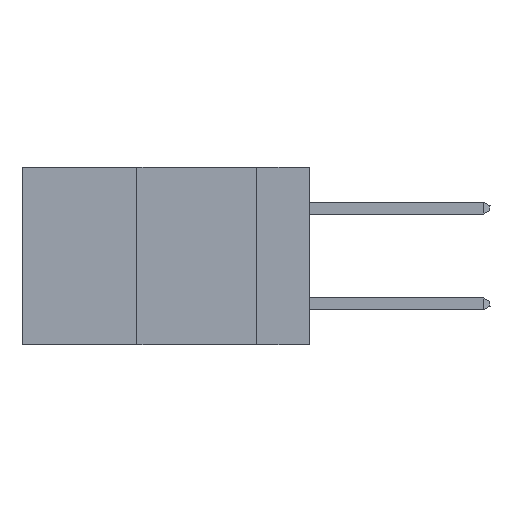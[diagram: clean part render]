
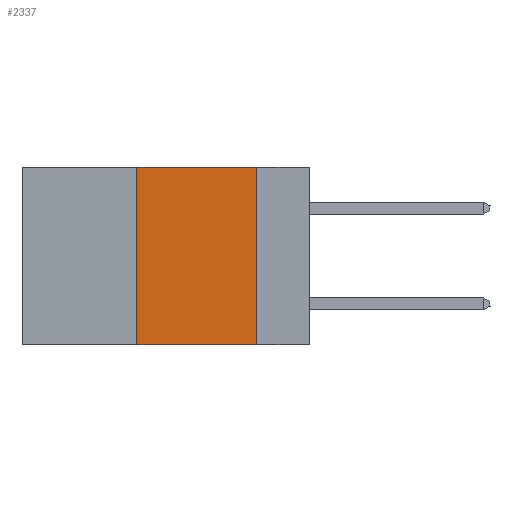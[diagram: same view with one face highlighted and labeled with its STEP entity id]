
A CAD part, left-side view. The second image highlights one B-rep face of the part: STEP entity #2337.
In plain terms, the highlighted planar face has unit normal (-1, 0, 0).
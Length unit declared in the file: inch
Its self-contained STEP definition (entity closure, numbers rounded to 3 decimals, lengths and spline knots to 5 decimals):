
#661 = CARTESIAN_POINT ( 'NONE',  ( 0., 0.36, -0.37 ) ) ;
#684 = VERTEX_POINT ( 'NONE', #33528 ) ;
#2337 = ADVANCED_FACE ( 'NONE', ( #24052 ), #7334, .F. ) ;
#2717 = CARTESIAN_POINT ( 'NONE',  ( 0., 0.6, 0. ) ) ;
#2844 = VECTOR ( 'NONE', #7003, 39.37008 ) ;
#3004 = EDGE_CURVE ( 'NONE', #35442, #684, #9142, .T. ) ;
#4611 = DIRECTION ( 'NONE',  ( 1., 0., 0. ) ) ;
#5510 = CARTESIAN_POINT ( 'NONE',  ( 0., 0.11, 0. ) ) ;
#5900 = EDGE_LOOP ( 'NONE', ( #15593, #10784, #30600, #32843 ) ) ;
#7003 = DIRECTION ( 'NONE',  ( 0., -1., 0. ) ) ;
#7334 = PLANE ( 'NONE',  #17374 ) ;
#9142 = LINE ( 'NONE', #5510, #30997 ) ;
#9614 = EDGE_CURVE ( 'NONE', #21436, #35442, #11652, .T. ) ;
#9817 = EDGE_CURVE ( 'NONE', #29942, #684, #22543, .T. ) ;
#10333 = VECTOR ( 'NONE', #11799, 39.37008 ) ;
#10784 = ORIENTED_EDGE ( 'NONE', *, *, #9614, .F. ) ;
#11652 = LINE ( 'NONE', #2717, #10333 ) ;
#11799 = DIRECTION ( 'NONE',  ( 0., -1., 0. ) ) ;
#13069 = DIRECTION ( 'NONE',  ( 0., 0., -1. ) ) ;
#15593 = ORIENTED_EDGE ( 'NONE', *, *, #3004, .F. ) ;
#16392 = CARTESIAN_POINT ( 'NONE',  ( 0., 0.11, 0. ) ) ;
#16436 = CARTESIAN_POINT ( 'NONE',  ( 0., 0.36, 0. ) ) ;
#17374 = AXIS2_PLACEMENT_3D ( 'NONE', #21380, #4611, #13069 ) ;
#18817 = CARTESIAN_POINT ( 'NONE',  ( 0., 0.36, 0. ) ) ;
#21380 = CARTESIAN_POINT ( 'NONE',  ( 0., 0.6, 0. ) ) ;
#21436 = VERTEX_POINT ( 'NONE', #18817 ) ;
#22543 = LINE ( 'NONE', #29394, #2844 ) ;
#24052 = FACE_OUTER_BOUND ( 'NONE', #5900, .T. ) ;
#24634 = DIRECTION ( 'NONE',  ( 0., 0., 1. ) ) ;
#24975 = DIRECTION ( 'NONE',  ( 0., 0., -1. ) ) ;
#25249 = EDGE_CURVE ( 'NONE', #29942, #21436, #26718, .T. ) ;
#26718 = LINE ( 'NONE', #16436, #28904 ) ;
#28904 = VECTOR ( 'NONE', #24634, 39.37008 ) ;
#29394 = CARTESIAN_POINT ( 'NONE',  ( 0., 0.6, -0.37 ) ) ;
#29942 = VERTEX_POINT ( 'NONE', #661 ) ;
#30600 = ORIENTED_EDGE ( 'NONE', *, *, #25249, .F. ) ;
#30997 = VECTOR ( 'NONE', #24975, 39.37008 ) ;
#32843 = ORIENTED_EDGE ( 'NONE', *, *, #9817, .T. ) ;
#33528 = CARTESIAN_POINT ( 'NONE',  ( 0., 0.11, -0.37 ) ) ;
#35442 = VERTEX_POINT ( 'NONE', #16392 ) ;
